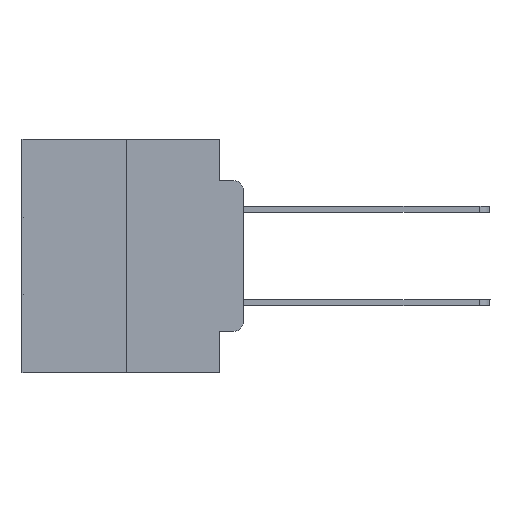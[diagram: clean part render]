
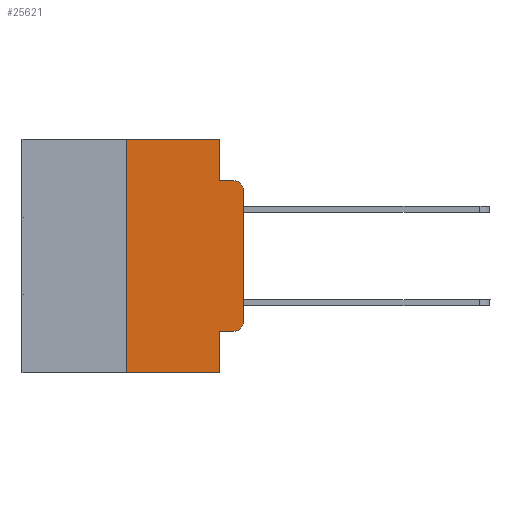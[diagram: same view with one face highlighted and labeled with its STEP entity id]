
A CAD part, left-side view. The second image highlights one B-rep face of the part: STEP entity #25621.
In plain terms, the highlighted planar face has unit normal (-1, 0, 0).
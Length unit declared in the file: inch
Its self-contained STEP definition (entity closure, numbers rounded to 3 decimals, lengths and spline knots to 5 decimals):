
#599 = CARTESIAN_POINT ( 'NONE',  ( 0., 0.051, 0. ) ) ;
#641 = LINE ( 'NONE', #22276, #26492 ) ;
#759 = DIRECTION ( 'NONE',  ( 0., -1., 0. ) ) ;
#1151 = VECTOR ( 'NONE', #19190, 39.37008 ) ;
#1421 = CARTESIAN_POINT ( 'NONE',  ( 0., 0.02, -0.1085 ) ) ;
#1499 = DIRECTION ( 'NONE',  ( 1., 0., 0. ) ) ;
#1681 = VECTOR ( 'NONE', #28393, 39.37008 ) ;
#2202 = EDGE_CURVE ( 'NONE', #3037, #12181, #21857, .T. ) ;
#2585 = VERTEX_POINT ( 'NONE', #10160 ) ;
#2659 = DIRECTION ( 'NONE',  ( 0., 0., 1. ) ) ;
#2749 = ORIENTED_EDGE ( 'NONE', *, *, #19047, .T. ) ;
#2916 = ORIENTED_EDGE ( 'NONE', *, *, #26739, .T. ) ;
#3037 = VERTEX_POINT ( 'NONE', #5749 ) ;
#3102 = CARTESIAN_POINT ( 'NONE',  ( 0., 0.051, -0.4115 ) ) ;
#3220 = VERTEX_POINT ( 'NONE', #10221 ) ;
#3408 = ORIENTED_EDGE ( 'NONE', *, *, #20160, .T. ) ;
#3595 = DIRECTION ( 'NONE',  ( 0., 0., -1. ) ) ;
#3675 = ORIENTED_EDGE ( 'NONE', *, *, #14690, .F. ) ;
#3731 = CARTESIAN_POINT ( 'NONE',  ( 0., 0.051, -0.4115 ) ) ;
#4768 = DIRECTION ( 'NONE',  ( 0., -1., 0. ) ) ;
#4840 = CIRCLE ( 'NONE', #12454, 0.02 ) ;
#4855 = CARTESIAN_POINT ( 'NONE',  ( 0., 0.25, 0. ) ) ;
#5346 = EDGE_LOOP ( 'NONE', ( #5870, #14755, #22228, #24522, #22057, #6038, #3408, #3675, #2749, #2916 ) ) ;
#5505 = EDGE_CURVE ( 'NONE', #12181, #18492, #17136, .T. ) ;
#5749 = CARTESIAN_POINT ( 'NONE',  ( 0., 0.25, -0.5 ) ) ;
#5870 = ORIENTED_EDGE ( 'NONE', *, *, #14248, .T. ) ;
#5997 = DIRECTION ( 'NONE',  ( 0., 0., -1. ) ) ;
#6038 = ORIENTED_EDGE ( 'NONE', *, *, #2202, .F. ) ;
#6638 = DIRECTION ( 'NONE',  ( -1., 0., 0. ) ) ;
#7193 = CARTESIAN_POINT ( 'NONE',  ( 0., 0.051, -0.0885 ) ) ;
#7603 = VECTOR ( 'NONE', #24604, 39.37008 ) ;
#8604 = CARTESIAN_POINT ( 'NONE',  ( 0., 0., -0.1085 ) ) ;
#9159 = CARTESIAN_POINT ( 'NONE',  ( 0., 0.02, -0.3915 ) ) ;
#9182 = LINE ( 'NONE', #21526, #1151 ) ;
#9211 = CARTESIAN_POINT ( 'NONE',  ( 0., 0.051, 0. ) ) ;
#9412 = CARTESIAN_POINT ( 'NONE',  ( 0., 0.02, -0.4115 ) ) ;
#9583 = CARTESIAN_POINT ( 'NONE',  ( 0., 0.25, 0. ) ) ;
#10160 = CARTESIAN_POINT ( 'NONE',  ( 0., 0.051, -0.0885 ) ) ;
#10221 = CARTESIAN_POINT ( 'NONE',  ( 0., 0.051, -0.5 ) ) ;
#10478 = CARTESIAN_POINT ( 'NONE',  ( 0., 0.473, 0. ) ) ;
#11064 = CARTESIAN_POINT ( 'NONE',  ( 0., 0., -0.3915 ) ) ;
#11198 = FACE_OUTER_BOUND ( 'NONE', #5346, .T. ) ;
#12181 = VERTEX_POINT ( 'NONE', #4855 ) ;
#12454 = AXIS2_PLACEMENT_3D ( 'NONE', #1421, #14607, #3595 ) ;
#12580 = VECTOR ( 'NONE', #21950, 39.37008 ) ;
#12881 = CARTESIAN_POINT ( 'NONE',  ( 0., 0.473, 0. ) ) ;
#12884 = LINE ( 'NONE', #7193, #27907 ) ;
#13100 = PLANE ( 'NONE',  #13508 ) ;
#13490 = VECTOR ( 'NONE', #2659, 39.37008 ) ;
#13508 = AXIS2_PLACEMENT_3D ( 'NONE', #10478, #1499, #5997 ) ;
#14248 = EDGE_CURVE ( 'NONE', #27979, #28593, #641, .T. ) ;
#14281 = AXIS2_PLACEMENT_3D ( 'NONE', #9159, #6638, #18056 ) ;
#14607 = DIRECTION ( 'NONE',  ( -1., 0., 0. ) ) ;
#14690 = EDGE_CURVE ( 'NONE', #24607, #3220, #26100, .T. ) ;
#14755 = ORIENTED_EDGE ( 'NONE', *, *, #27551, .T. ) ;
#16155 = VERTEX_POINT ( 'NONE', #9412 ) ;
#17136 = LINE ( 'NONE', #12881, #12580 ) ;
#17981 = LINE ( 'NONE', #3102, #21099 ) ;
#18056 = DIRECTION ( 'NONE',  ( 0., 0., -1. ) ) ;
#18492 = VERTEX_POINT ( 'NONE', #599 ) ;
#19047 = EDGE_CURVE ( 'NONE', #24607, #16155, #17981, .T. ) ;
#19190 = DIRECTION ( 'NONE',  ( 0., -1., 0. ) ) ;
#20160 = EDGE_CURVE ( 'NONE', #3037, #3220, #9182, .T. ) ;
#21099 = VECTOR ( 'NONE', #759, 39.37008 ) ;
#21265 = VERTEX_POINT ( 'NONE', #25256 ) ;
#21526 = CARTESIAN_POINT ( 'NONE',  ( 0., 0.473, -0.5 ) ) ;
#21659 = CARTESIAN_POINT ( 'NONE',  ( 0., 0.051, 0. ) ) ;
#21857 = LINE ( 'NONE', #9583, #13490 ) ;
#21950 = DIRECTION ( 'NONE',  ( 0., -1., 0. ) ) ;
#22057 = ORIENTED_EDGE ( 'NONE', *, *, #5505, .F. ) ;
#22228 = ORIENTED_EDGE ( 'NONE', *, *, #27412, .F. ) ;
#22276 = CARTESIAN_POINT ( 'NONE',  ( 0., 0., 0. ) ) ;
#23643 = LINE ( 'NONE', #9211, #7603 ) ;
#24522 = ORIENTED_EDGE ( 'NONE', *, *, #27945, .F. ) ;
#24601 = DIRECTION ( 'NONE',  ( 0., 0., 1. ) ) ;
#24604 = DIRECTION ( 'NONE',  ( 0., 0., -1. ) ) ;
#24607 = VERTEX_POINT ( 'NONE', #3731 ) ;
#25256 = CARTESIAN_POINT ( 'NONE',  ( 0., 0.02, -0.0885 ) ) ;
#25621 = ADVANCED_FACE ( 'NONE', ( #11198 ), #13100, .F. ) ;
#26100 = LINE ( 'NONE', #21659, #1681 ) ;
#26492 = VECTOR ( 'NONE', #24601, 39.37008 ) ;
#26739 = EDGE_CURVE ( 'NONE', #16155, #27979, #27902, .T. ) ;
#27412 = EDGE_CURVE ( 'NONE', #2585, #21265, #12884, .T. ) ;
#27551 = EDGE_CURVE ( 'NONE', #28593, #21265, #4840, .T. ) ;
#27902 = CIRCLE ( 'NONE', #14281, 0.02 ) ;
#27907 = VECTOR ( 'NONE', #4768, 39.37008 ) ;
#27945 = EDGE_CURVE ( 'NONE', #18492, #2585, #23643, .T. ) ;
#27979 = VERTEX_POINT ( 'NONE', #11064 ) ;
#28393 = DIRECTION ( 'NONE',  ( 0., 0., -1. ) ) ;
#28593 = VERTEX_POINT ( 'NONE', #8604 ) ;
